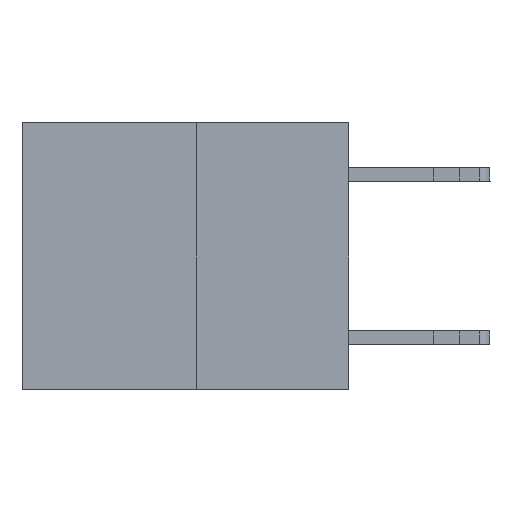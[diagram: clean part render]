
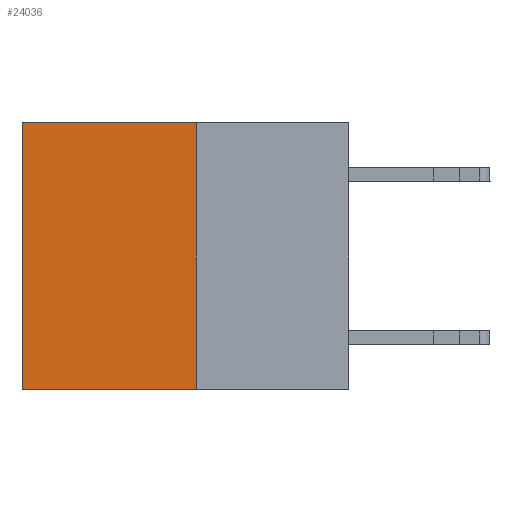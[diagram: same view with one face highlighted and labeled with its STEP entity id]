
A CAD part, left-side view. The second image highlights one B-rep face of the part: STEP entity #24036.
In plain terms, the highlighted planar face has unit normal (-1, 0, 0).
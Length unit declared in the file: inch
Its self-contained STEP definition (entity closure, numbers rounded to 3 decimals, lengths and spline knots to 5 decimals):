
#1358 = DIRECTION ( 'NONE',  ( 0., 0., -1. ) ) ;
#1779 = CARTESIAN_POINT ( 'NONE',  ( 0.3165, 0.28, -0.49 ) ) ;
#3684 = FACE_OUTER_BOUND ( 'NONE', #4207, .T. ) ;
#3829 = CARTESIAN_POINT ( 'NONE',  ( 0.3165, 0.6, 0. ) ) ;
#4207 = EDGE_LOOP ( 'NONE', ( #20912, #21611, #4872, #16349 ) ) ;
#4580 = VERTEX_POINT ( 'NONE', #16256 ) ;
#4872 = ORIENTED_EDGE ( 'NONE', *, *, #18533, .F. ) ;
#6501 = EDGE_CURVE ( 'NONE', #18292, #4580, #11155, .T. ) ;
#7349 = LINE ( 'NONE', #18664, #24878 ) ;
#7646 = CARTESIAN_POINT ( 'NONE',  ( 0.3165, 0.28, -0.49 ) ) ;
#7900 = CARTESIAN_POINT ( 'NONE',  ( 0.3165, 0.28, 0. ) ) ;
#8350 = EDGE_CURVE ( 'NONE', #18585, #4580, #19901, .T. ) ;
#11155 = LINE ( 'NONE', #1779, #15852 ) ;
#12535 = CARTESIAN_POINT ( 'NONE',  ( 0.3165, 0.6, -0.49 ) ) ;
#13640 = DIRECTION ( 'NONE',  ( 0., 0., -1. ) ) ;
#13734 = CARTESIAN_POINT ( 'NONE',  ( 0.3165, 0.28, -0.49 ) ) ;
#14729 = EDGE_CURVE ( 'NONE', #24911, #18585, #7349, .T. ) ;
#14830 = VECTOR ( 'NONE', #23201, 39.37008 ) ;
#15852 = VECTOR ( 'NONE', #21221, 39.37008 ) ;
#15994 = PLANE ( 'NONE',  #19747 ) ;
#16256 = CARTESIAN_POINT ( 'NONE',  ( 0.3165, 0.6, -0.49 ) ) ;
#16349 = ORIENTED_EDGE ( 'NONE', *, *, #14729, .T. ) ;
#18292 = VERTEX_POINT ( 'NONE', #21857 ) ;
#18297 = VECTOR ( 'NONE', #1358, 39.37008 ) ;
#18533 = EDGE_CURVE ( 'NONE', #24911, #18292, #24009, .T. ) ;
#18585 = VERTEX_POINT ( 'NONE', #3829 ) ;
#18664 = CARTESIAN_POINT ( 'NONE',  ( 0.3165, 0.28, 0. ) ) ;
#19747 = AXIS2_PLACEMENT_3D ( 'NONE', #13734, #24384, #13640 ) ;
#19901 = LINE ( 'NONE', #12535, #14830 ) ;
#20813 = DIRECTION ( 'NONE',  ( 0., 1., 0. ) ) ;
#20912 = ORIENTED_EDGE ( 'NONE', *, *, #8350, .T. ) ;
#21221 = DIRECTION ( 'NONE',  ( 0., 1., 0. ) ) ;
#21611 = ORIENTED_EDGE ( 'NONE', *, *, #6501, .F. ) ;
#21857 = CARTESIAN_POINT ( 'NONE',  ( 0.3165, 0.28, -0.49 ) ) ;
#23201 = DIRECTION ( 'NONE',  ( 0., 0., -1. ) ) ;
#24009 = LINE ( 'NONE', #7646, #18297 ) ;
#24036 = ADVANCED_FACE ( 'NONE', ( #3684 ), #15994, .F. ) ;
#24384 = DIRECTION ( 'NONE',  ( 1., 0., 0. ) ) ;
#24878 = VECTOR ( 'NONE', #20813, 39.37008 ) ;
#24911 = VERTEX_POINT ( 'NONE', #7900 ) ;
